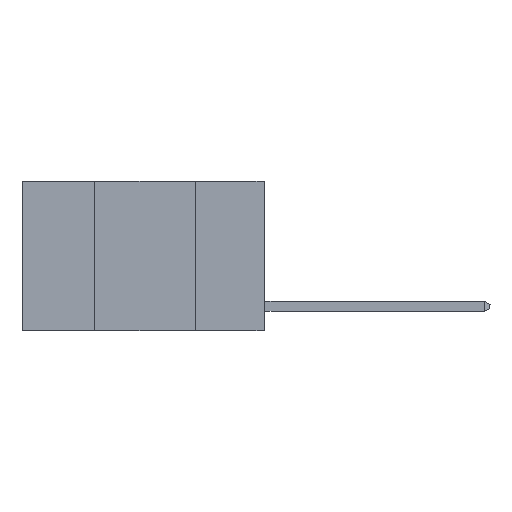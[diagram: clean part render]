
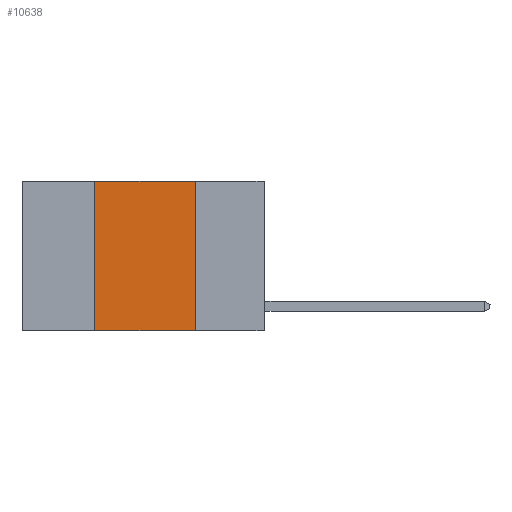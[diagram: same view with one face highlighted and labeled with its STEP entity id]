
A CAD part, left-side view. The second image highlights one B-rep face of the part: STEP entity #10638.
In plain terms, the highlighted planar face has unit normal (-1, 0, 0).
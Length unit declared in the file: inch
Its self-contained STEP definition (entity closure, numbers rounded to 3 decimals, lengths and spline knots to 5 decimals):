
#348 = PLANE ( 'NONE',  #3829 ) ;
#393 = VECTOR ( 'NONE', #4847, 39.37008 ) ;
#426 = DIRECTION ( 'NONE',  ( 1., 0., 0. ) ) ;
#539 = CARTESIAN_POINT ( 'NONE',  ( 0., 0.17, -0.37 ) ) ;
#713 = CARTESIAN_POINT ( 'NONE',  ( 0., 0.42, 0. ) ) ;
#949 = VECTOR ( 'NONE', #5434, 39.37008 ) ;
#1438 = CARTESIAN_POINT ( 'NONE',  ( 0., 0.6, -0.37 ) ) ;
#2390 = EDGE_LOOP ( 'NONE', ( #7852, #13065, #9733, #2754 ) ) ;
#2754 = ORIENTED_EDGE ( 'NONE', *, *, #2974, .T. ) ;
#2974 = EDGE_CURVE ( 'NONE', #14042, #6471, #12643, .T. ) ;
#3009 = CARTESIAN_POINT ( 'NONE',  ( 0., 0.6, 0. ) ) ;
#3547 = DIRECTION ( 'NONE',  ( 0., 0., -1. ) ) ;
#3829 = AXIS2_PLACEMENT_3D ( 'NONE', #4952, #426, #3547 ) ;
#4275 = EDGE_CURVE ( 'NONE', #10199, #6471, #5292, .T. ) ;
#4370 = CARTESIAN_POINT ( 'NONE',  ( 0., 0.42, -0.37 ) ) ;
#4847 = DIRECTION ( 'NONE',  ( 0., -1., 0. ) ) ;
#4952 = CARTESIAN_POINT ( 'NONE',  ( 0., 0.6, 0. ) ) ;
#5292 = LINE ( 'NONE', #11150, #949 ) ;
#5434 = DIRECTION ( 'NONE',  ( 0., 0., -1. ) ) ;
#6465 = DIRECTION ( 'NONE',  ( 0., -1., 0. ) ) ;
#6471 = VERTEX_POINT ( 'NONE', #539 ) ;
#6542 = DIRECTION ( 'NONE',  ( 0., 0., 1. ) ) ;
#6818 = VECTOR ( 'NONE', #6465, 39.37008 ) ;
#7013 = VERTEX_POINT ( 'NONE', #713 ) ;
#7852 = ORIENTED_EDGE ( 'NONE', *, *, #4275, .F. ) ;
#7861 = CARTESIAN_POINT ( 'NONE',  ( 0., 0.42, 0. ) ) ;
#8764 = LINE ( 'NONE', #7861, #9904 ) ;
#9002 = EDGE_CURVE ( 'NONE', #7013, #10199, #13098, .T. ) ;
#9212 = CARTESIAN_POINT ( 'NONE',  ( 0., 0.17, 0. ) ) ;
#9733 = ORIENTED_EDGE ( 'NONE', *, *, #12002, .F. ) ;
#9904 = VECTOR ( 'NONE', #6542, 39.37008 ) ;
#10199 = VERTEX_POINT ( 'NONE', #9212 ) ;
#10638 = ADVANCED_FACE ( 'NONE', ( #11483 ), #348, .F. ) ;
#11150 = CARTESIAN_POINT ( 'NONE',  ( 0., 0.17, 0. ) ) ;
#11483 = FACE_OUTER_BOUND ( 'NONE', #2390, .T. ) ;
#12002 = EDGE_CURVE ( 'NONE', #14042, #7013, #8764, .T. ) ;
#12643 = LINE ( 'NONE', #1438, #393 ) ;
#13065 = ORIENTED_EDGE ( 'NONE', *, *, #9002, .F. ) ;
#13098 = LINE ( 'NONE', #3009, #6818 ) ;
#14042 = VERTEX_POINT ( 'NONE', #4370 ) ;
